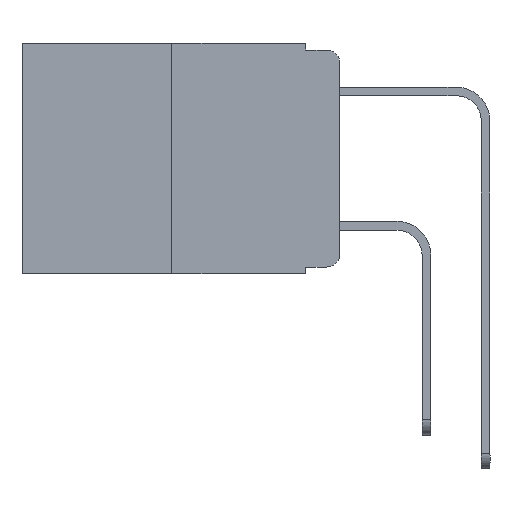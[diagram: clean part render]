
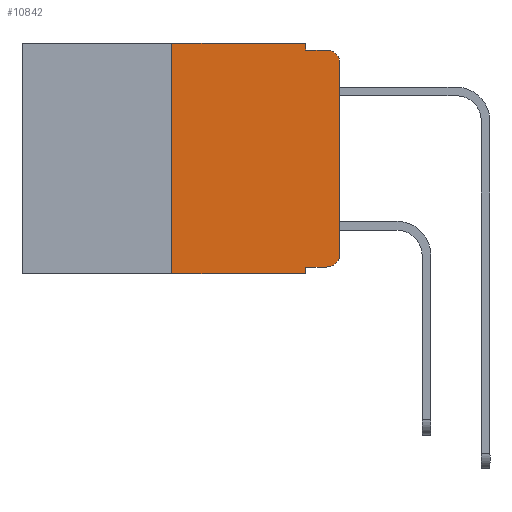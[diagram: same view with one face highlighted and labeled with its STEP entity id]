
A CAD part, left-side view. The second image highlights one B-rep face of the part: STEP entity #10842.
In plain terms, the highlighted planar face has unit normal (-1, 0, 0).
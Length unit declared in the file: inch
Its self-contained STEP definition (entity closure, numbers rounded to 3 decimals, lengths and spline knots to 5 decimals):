
#107 = VECTOR ( 'NONE', #3696, 39.37008 ) ;
#1258 = DIRECTION ( 'NONE',  ( 0., -1., 0. ) ) ;
#1299 = DIRECTION ( 'NONE',  ( 0., 0., 1. ) ) ;
#1535 = CARTESIAN_POINT ( 'NONE',  ( 0., 0.473, 0. ) ) ;
#1821 = CIRCLE ( 'NONE', #11447, 0.02 ) ;
#1996 = EDGE_CURVE ( 'NONE', #8028, #13031, #3372, .T. ) ;
#2484 = EDGE_CURVE ( 'NONE', #5265, #18714, #23588, .T. ) ;
#2515 = LINE ( 'NONE', #18583, #19091 ) ;
#2894 = CARTESIAN_POINT ( 'NONE',  ( 0., 0.051, 0. ) ) ;
#3372 = LINE ( 'NONE', #9961, #26622 ) ;
#3696 = DIRECTION ( 'NONE',  ( 0., 0., 1. ) ) ;
#3890 = DIRECTION ( 'NONE',  ( 0., -1., 0. ) ) ;
#4290 = DIRECTION ( 'NONE',  ( 0., -1., 0. ) ) ;
#5265 = VERTEX_POINT ( 'NONE', #10930 ) ;
#6294 = VECTOR ( 'NONE', #12101, 39.37008 ) ;
#6320 = ORIENTED_EDGE ( 'NONE', *, *, #19065, .F. ) ;
#6570 = ORIENTED_EDGE ( 'NONE', *, *, #1996, .F. ) ;
#6721 = DIRECTION ( 'NONE',  ( -1., 0., 0. ) ) ;
#7008 = ORIENTED_EDGE ( 'NONE', *, *, #2484, .T. ) ;
#7935 = CARTESIAN_POINT ( 'NONE',  ( 0., 0.051, -0.01 ) ) ;
#8028 = VERTEX_POINT ( 'NONE', #2894 ) ;
#8404 = CARTESIAN_POINT ( 'NONE',  ( 0., 0.051, -0.333 ) ) ;
#8583 = EDGE_CURVE ( 'NONE', #5265, #17918, #10157, .T. ) ;
#8834 = EDGE_CURVE ( 'NONE', #18110, #12754, #18102, .T. ) ;
#9220 = ORIENTED_EDGE ( 'NONE', *, *, #22904, .T. ) ;
#9286 = CARTESIAN_POINT ( 'NONE',  ( 0., 0.051, -0.333 ) ) ;
#9941 = LINE ( 'NONE', #14545, #6294 ) ;
#9961 = CARTESIAN_POINT ( 'NONE',  ( 0., 0.051, 0. ) ) ;
#10063 = LINE ( 'NONE', #7935, #16687 ) ;
#10157 = LINE ( 'NONE', #23431, #107 ) ;
#10162 = ORIENTED_EDGE ( 'NONE', *, *, #8583, .F. ) ;
#10189 = ORIENTED_EDGE ( 'NONE', *, *, #8834, .T. ) ;
#10842 = ADVANCED_FACE ( 'NONE', ( #17508 ), #28496, .F. ) ;
#10930 = CARTESIAN_POINT ( 'NONE',  ( 0., 0.25, -0.343 ) ) ;
#10951 = CARTESIAN_POINT ( 'NONE',  ( 0., 0.051, -0.343 ) ) ;
#10984 = CARTESIAN_POINT ( 'NONE',  ( 0., 0., -0.313 ) ) ;
#11197 = LINE ( 'NONE', #13512, #27584 ) ;
#11447 = AXIS2_PLACEMENT_3D ( 'NONE', #12514, #25777, #17261 ) ;
#12101 = DIRECTION ( 'NONE',  ( 0., -1., 0. ) ) ;
#12268 = DIRECTION ( 'NONE',  ( 0., 0., -1. ) ) ;
#12514 = CARTESIAN_POINT ( 'NONE',  ( 0., 0.02, -0.03 ) ) ;
#12716 = AXIS2_PLACEMENT_3D ( 'NONE', #1535, #17081, #15205 ) ;
#12731 = EDGE_CURVE ( 'NONE', #21476, #18110, #28171, .T. ) ;
#12754 = VERTEX_POINT ( 'NONE', #10984 ) ;
#12877 = ORIENTED_EDGE ( 'NONE', *, *, #26169, .F. ) ;
#13031 = VERTEX_POINT ( 'NONE', #25118 ) ;
#13044 = CARTESIAN_POINT ( 'NONE',  ( 0., 0.473, -0.343 ) ) ;
#13512 = CARTESIAN_POINT ( 'NONE',  ( 0., 0.051, 0. ) ) ;
#13518 = EDGE_CURVE ( 'NONE', #14447, #23775, #1821, .T. ) ;
#13618 = EDGE_CURVE ( 'NONE', #21476, #18714, #11197, .T. ) ;
#14052 = CARTESIAN_POINT ( 'NONE',  ( 0., 0.02, -0.01 ) ) ;
#14447 = VERTEX_POINT ( 'NONE', #20651 ) ;
#14545 = CARTESIAN_POINT ( 'NONE',  ( 0., 0.473, 0. ) ) ;
#15111 = VECTOR ( 'NONE', #1258, 39.37008 ) ;
#15205 = DIRECTION ( 'NONE',  ( 0., 0., -1. ) ) ;
#16687 = VECTOR ( 'NONE', #3890, 39.37008 ) ;
#17081 = DIRECTION ( 'NONE',  ( 1., 0., 0. ) ) ;
#17261 = DIRECTION ( 'NONE',  ( 0., 0., -1. ) ) ;
#17501 = DIRECTION ( 'NONE',  ( 0., 0., -1. ) ) ;
#17508 = FACE_OUTER_BOUND ( 'NONE', #21773, .T. ) ;
#17918 = VERTEX_POINT ( 'NONE', #22206 ) ;
#18102 = CIRCLE ( 'NONE', #19936, 0.02 ) ;
#18110 = VERTEX_POINT ( 'NONE', #18137 ) ;
#18137 = CARTESIAN_POINT ( 'NONE',  ( 0., 0.02, -0.333 ) ) ;
#18465 = DIRECTION ( 'NONE',  ( 0., 0., -1. ) ) ;
#18583 = CARTESIAN_POINT ( 'NONE',  ( 0., 0., 0. ) ) ;
#18714 = VERTEX_POINT ( 'NONE', #10951 ) ;
#19065 = EDGE_CURVE ( 'NONE', #13031, #23775, #10063, .T. ) ;
#19091 = VECTOR ( 'NONE', #1299, 39.37008 ) ;
#19936 = AXIS2_PLACEMENT_3D ( 'NONE', #26456, #6721, #17501 ) ;
#20651 = CARTESIAN_POINT ( 'NONE',  ( 0., 0., -0.03 ) ) ;
#20736 = ORIENTED_EDGE ( 'NONE', *, *, #12731, .T. ) ;
#21476 = VERTEX_POINT ( 'NONE', #9286 ) ;
#21773 = EDGE_LOOP ( 'NONE', ( #9220, #28004, #6320, #6570, #12877, #10162, #7008, #25616, #20736, #10189 ) ) ;
#22206 = CARTESIAN_POINT ( 'NONE',  ( 0., 0.25, 0. ) ) ;
#22904 = EDGE_CURVE ( 'NONE', #12754, #14447, #2515, .T. ) ;
#23431 = CARTESIAN_POINT ( 'NONE',  ( 0., 0.25, 0. ) ) ;
#23588 = LINE ( 'NONE', #13044, #28030 ) ;
#23775 = VERTEX_POINT ( 'NONE', #14052 ) ;
#25118 = CARTESIAN_POINT ( 'NONE',  ( 0., 0.051, -0.01 ) ) ;
#25616 = ORIENTED_EDGE ( 'NONE', *, *, #13618, .F. ) ;
#25777 = DIRECTION ( 'NONE',  ( -1., 0., 0. ) ) ;
#26169 = EDGE_CURVE ( 'NONE', #17918, #8028, #9941, .T. ) ;
#26456 = CARTESIAN_POINT ( 'NONE',  ( 0., 0.02, -0.313 ) ) ;
#26622 = VECTOR ( 'NONE', #12268, 39.37008 ) ;
#27584 = VECTOR ( 'NONE', #18465, 39.37008 ) ;
#28004 = ORIENTED_EDGE ( 'NONE', *, *, #13518, .T. ) ;
#28030 = VECTOR ( 'NONE', #4290, 39.37008 ) ;
#28171 = LINE ( 'NONE', #8404, #15111 ) ;
#28496 = PLANE ( 'NONE',  #12716 ) ;
